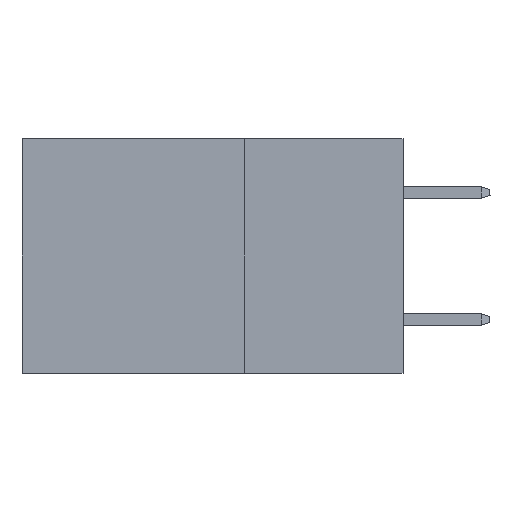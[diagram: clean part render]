
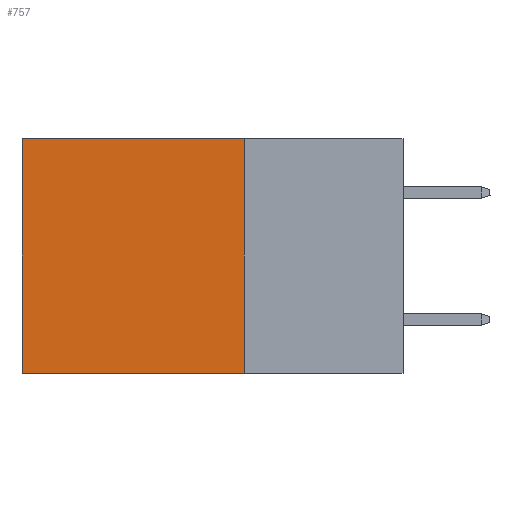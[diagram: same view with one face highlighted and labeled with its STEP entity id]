
A CAD part, left-side view. The second image highlights one B-rep face of the part: STEP entity #757.
In plain terms, the highlighted planar face has unit normal (-1, 0, 0).
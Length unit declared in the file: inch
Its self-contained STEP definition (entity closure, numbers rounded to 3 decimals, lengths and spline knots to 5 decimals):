
#740 = ORIENTED_EDGE ( 'NONE', *, *, #12642, .F. ) ;
#757 = ADVANCED_FACE ( 'NONE', ( #17718 ), #4054, .F. ) ;
#2446 = CARTESIAN_POINT ( 'NONE',  ( 0.2875, 0.25, 0. ) ) ;
#3481 = ORIENTED_EDGE ( 'NONE', *, *, #4661, .T. ) ;
#4054 = PLANE ( 'NONE',  #4152 ) ;
#4152 = AXIS2_PLACEMENT_3D ( 'NONE', #2446, #5249, #9292 ) ;
#4661 = EDGE_CURVE ( 'NONE', #16167, #15850, #8489, .T. ) ;
#5249 = DIRECTION ( 'NONE',  ( 1., 0., 0. ) ) ;
#5355 = VERTEX_POINT ( 'NONE', #7310 ) ;
#5564 = CARTESIAN_POINT ( 'NONE',  ( 0.2875, 0.25, -0.37 ) ) ;
#5811 = CARTESIAN_POINT ( 'NONE',  ( 0.2875, 0.25, 0. ) ) ;
#6652 = VECTOR ( 'NONE', #12230, 39.37008 ) ;
#7310 = CARTESIAN_POINT ( 'NONE',  ( 0.2875, 0.6, -0.37 ) ) ;
#7749 = LINE ( 'NONE', #11940, #14176 ) ;
#8358 = DIRECTION ( 'NONE',  ( 0., 0., -1. ) ) ;
#8489 = LINE ( 'NONE', #5811, #17836 ) ;
#8521 = LINE ( 'NONE', #11320, #17366 ) ;
#9292 = DIRECTION ( 'NONE',  ( 0., 0., -1. ) ) ;
#9698 = LINE ( 'NONE', #5564, #6652 ) ;
#10049 = VERTEX_POINT ( 'NONE', #17707 ) ;
#10849 = ORIENTED_EDGE ( 'NONE', *, *, #11961, .T. ) ;
#11320 = CARTESIAN_POINT ( 'NONE',  ( 0.2875, 0.6, 0. ) ) ;
#11940 = CARTESIAN_POINT ( 'NONE',  ( 0.2875, 0.25, 0. ) ) ;
#11961 = EDGE_CURVE ( 'NONE', #15850, #5355, #8521, .T. ) ;
#12230 = DIRECTION ( 'NONE',  ( 0., 1., 0. ) ) ;
#12642 = EDGE_CURVE ( 'NONE', #16167, #10049, #7749, .T. ) ;
#14176 = VECTOR ( 'NONE', #8358, 39.37008 ) ;
#14306 = DIRECTION ( 'NONE',  ( 0., 0., -1. ) ) ;
#14799 = CARTESIAN_POINT ( 'NONE',  ( 0.2875, 0.25, 0. ) ) ;
#14936 = EDGE_CURVE ( 'NONE', #10049, #5355, #9698, .T. ) ;
#15850 = VERTEX_POINT ( 'NONE', #16818 ) ;
#16167 = VERTEX_POINT ( 'NONE', #14799 ) ;
#16818 = CARTESIAN_POINT ( 'NONE',  ( 0.2875, 0.6, 0. ) ) ;
#17000 = EDGE_LOOP ( 'NONE', ( #10849, #17900, #740, #3481 ) ) ;
#17014 = DIRECTION ( 'NONE',  ( 0., 1., 0. ) ) ;
#17366 = VECTOR ( 'NONE', #14306, 39.37008 ) ;
#17707 = CARTESIAN_POINT ( 'NONE',  ( 0.2875, 0.25, -0.37 ) ) ;
#17718 = FACE_OUTER_BOUND ( 'NONE', #17000, .T. ) ;
#17836 = VECTOR ( 'NONE', #17014, 39.37008 ) ;
#17900 = ORIENTED_EDGE ( 'NONE', *, *, #14936, .F. ) ;
